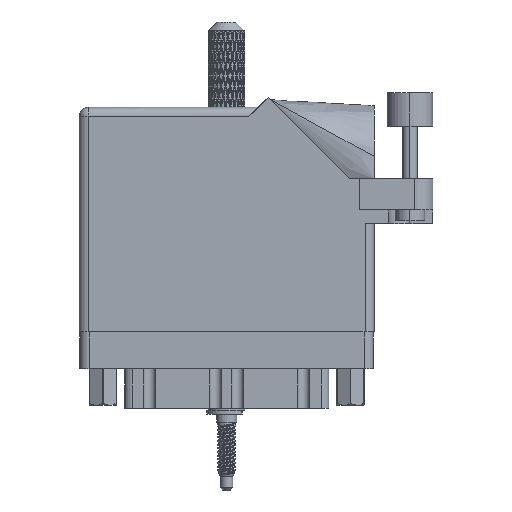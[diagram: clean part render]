
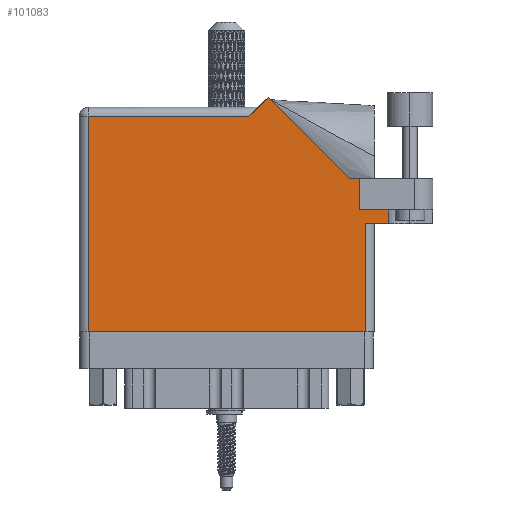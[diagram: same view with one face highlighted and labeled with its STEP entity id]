
A CAD part, front view. The second image highlights one B-rep face of the part: STEP entity #101083.
In plain terms, the highlighted face is planar.
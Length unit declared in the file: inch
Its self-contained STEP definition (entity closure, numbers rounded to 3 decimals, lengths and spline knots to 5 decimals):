
#764 = ORIENTED_EDGE ( 'NONE', *, *, #93199, .F. ) ;
#1494 = CARTESIAN_POINT ( 'NONE',  ( 0.062, 0., 0. ) ) ;
#5880 = DIRECTION ( 'NONE',  ( -1., 0., 0. ) ) ;
#8115 = ORIENTED_EDGE ( 'NONE', *, *, #74659, .T. ) ;
#10553 = CARTESIAN_POINT ( 'NONE',  ( 2.1115, 0.737, 0. ) ) ;
#10583 = VECTOR ( 'NONE', #10934, 39.37008 ) ;
#10934 = DIRECTION ( 'NONE',  ( 0., -1., 0. ) ) ;
#11982 = VERTEX_POINT ( 'NONE', #92862 ) ;
#13901 = DIRECTION ( 'NONE',  ( 1., 0., 0. ) ) ;
#15610 = VECTOR ( 'NONE', #15700, 39.37008 ) ;
#15700 = DIRECTION ( 'NONE',  ( -0.707, 0.707, 0. ) ) ;
#16142 = EDGE_CURVE ( 'NONE', #69696, #36570, #74704, .T. ) ;
#17372 = EDGE_CURVE ( 'NONE', #57398, #100621, #43704, .T. ) ;
#19483 = DIRECTION ( 'NONE',  ( -1., 0., 0. ) ) ;
#20174 = VERTEX_POINT ( 'NONE', #97081 ) ;
#22118 = CARTESIAN_POINT ( 'NONE',  ( 0.062, 0., 0. ) ) ;
#22520 = LINE ( 'NONE', #57601, #79626 ) ;
#24242 = EDGE_CURVE ( 'NONE', #81942, #102610, #106608, .T. ) ;
#27284 = DIRECTION ( 'NONE',  ( 0., -1., 0. ) ) ;
#28101 = CARTESIAN_POINT ( 'NONE',  ( 2.41, 1.044, 0. ) ) ;
#30601 = CARTESIAN_POINT ( 'NONE',  ( 1.91, 0.831, 0. ) ) ;
#32043 = ORIENTED_EDGE ( 'NONE', *, *, #16142, .T. ) ;
#32108 = EDGE_CURVE ( 'NONE', #36570, #81942, #65064, .T. ) ;
#33150 = AXIS2_PLACEMENT_3D ( 'NONE', #111329, #84917, #95279 ) ;
#36570 = VERTEX_POINT ( 'NONE', #84374 ) ;
#36747 = LINE ( 'NONE', #28101, #78238 ) ;
#38378 = ORIENTED_EDGE ( 'NONE', *, *, #86738, .F. ) ;
#40867 = CARTESIAN_POINT ( 'NONE',  ( 0., 1.468, 0. ) ) ;
#41526 = EDGE_LOOP ( 'NONE', ( #105941, #44499, #101186, #764, #38378, #53182, #8115, #90428, #32043, #53290, #87346 ) ) ;
#42484 = CARTESIAN_POINT ( 'NONE',  ( 1.91, 0.831, 0. ) ) ;
#43324 = VERTEX_POINT ( 'NONE', #94800 ) ;
#43704 = LINE ( 'NONE', #113252, #76299 ) ;
#44499 = ORIENTED_EDGE ( 'NONE', *, *, #60868, .T. ) ;
#48830 = CARTESIAN_POINT ( 'NONE',  ( 1.217, 1.53, 0. ) ) ;
#48988 = DIRECTION ( 'NONE',  ( 1., 0., 0. ) ) ;
#49410 = LINE ( 'NONE', #42484, #67772 ) ;
#49412 = VECTOR ( 'NONE', #59577, 39.37008 ) ;
#51460 = VERTEX_POINT ( 'NONE', #56876 ) ;
#53182 = ORIENTED_EDGE ( 'NONE', *, *, #87078, .T. ) ;
#53290 = ORIENTED_EDGE ( 'NONE', *, *, #32108, .T. ) ;
#56044 = CARTESIAN_POINT ( 'NONE',  ( 1.28771, 1.60071, 0. ) ) ;
#56068 = CARTESIAN_POINT ( 'NONE',  ( 2.1115, 0.831, 0. ) ) ;
#56876 = CARTESIAN_POINT ( 'NONE',  ( 1.91, 1.044, 0. ) ) ;
#57398 = VERTEX_POINT ( 'NONE', #92781 ) ;
#57601 = CARTESIAN_POINT ( 'NONE',  ( 0., 0., 0. ) ) ;
#58112 = VECTOR ( 'NONE', #27284, 39.37008 ) ;
#59577 = DIRECTION ( 'NONE',  ( 0., 1., 0. ) ) ;
#60221 = FACE_OUTER_BOUND ( 'NONE', #41526, .T. ) ;
#60868 = EDGE_CURVE ( 'NONE', #20174, #57398, #77374, .T. ) ;
#63235 = VECTOR ( 'NONE', #90836, 39.37008 ) ;
#63322 = EDGE_CURVE ( 'NONE', #102610, #20174, #22520, .T. ) ;
#65064 = LINE ( 'NONE', #40867, #99186 ) ;
#66901 = EDGE_CURVE ( 'NONE', #11982, #69696, #110541, .T. ) ;
#67772 = VECTOR ( 'NONE', #68947, 39.37008 ) ;
#68947 = DIRECTION ( 'NONE',  ( 0., 1., 0. ) ) ;
#69696 = VERTEX_POINT ( 'NONE', #56044 ) ;
#74309 = LINE ( 'NONE', #30601, #75006 ) ;
#74659 = EDGE_CURVE ( 'NONE', #51460, #11982, #36747, .T. ) ;
#74704 = LINE ( 'NONE', #48830, #63235 ) ;
#75006 = VECTOR ( 'NONE', #48988, 39.37008 ) ;
#75577 = CARTESIAN_POINT ( 'NONE',  ( 0.062, 1.468, 0. ) ) ;
#76299 = VECTOR ( 'NONE', #86272, 39.37008 ) ;
#77374 = LINE ( 'NONE', #95204, #49412 ) ;
#77448 = PLANE ( 'NONE',  #33150 ) ;
#78238 = VECTOR ( 'NONE', #19483, 39.37008 ) ;
#79626 = VECTOR ( 'NONE', #13901, 39.37008 ) ;
#81942 = VERTEX_POINT ( 'NONE', #75577 ) ;
#84374 = CARTESIAN_POINT ( 'NONE',  ( 1.155, 1.468, 0. ) ) ;
#84917 = DIRECTION ( 'NONE',  ( 0., 0., -1. ) ) ;
#86272 = DIRECTION ( 'NONE',  ( 1., 0., 0. ) ) ;
#86738 = EDGE_CURVE ( 'NONE', #43324, #110630, #74309, .T. ) ;
#87078 = EDGE_CURVE ( 'NONE', #43324, #51460, #49410, .T. ) ;
#87346 = ORIENTED_EDGE ( 'NONE', *, *, #24242, .T. ) ;
#89661 = LINE ( 'NONE', #98292, #10583 ) ;
#90428 = ORIENTED_EDGE ( 'NONE', *, *, #66901, .T. ) ;
#90836 = DIRECTION ( 'NONE',  ( -0.707, -0.707, 0. ) ) ;
#92781 = CARTESIAN_POINT ( 'NONE',  ( 1.948, 0.737, 0. ) ) ;
#92862 = CARTESIAN_POINT ( 'NONE',  ( 1.84442, 1.044, 0. ) ) ;
#93199 = EDGE_CURVE ( 'NONE', #110630, #100621, #89661, .T. ) ;
#94800 = CARTESIAN_POINT ( 'NONE',  ( 1.91, 0.831, 0. ) ) ;
#95204 = CARTESIAN_POINT ( 'NONE',  ( 1.948, 0.737, 0. ) ) ;
#95279 = DIRECTION ( 'NONE',  ( -1., 0., 0. ) ) ;
#97081 = CARTESIAN_POINT ( 'NONE',  ( 1.948, 0., 0. ) ) ;
#98292 = CARTESIAN_POINT ( 'NONE',  ( 2.1115, 1.16177, 0. ) ) ;
#99186 = VECTOR ( 'NONE', #5880, 39.37008 ) ;
#100621 = VERTEX_POINT ( 'NONE', #10553 ) ;
#101083 = ADVANCED_FACE ( 'NONE', ( #60221 ), #77448, .F. ) ;
#101186 = ORIENTED_EDGE ( 'NONE', *, *, #17372, .T. ) ;
#102508 = CARTESIAN_POINT ( 'NONE',  ( 1.84442, 1.044, 0. ) ) ;
#102610 = VERTEX_POINT ( 'NONE', #22118 ) ;
#105941 = ORIENTED_EDGE ( 'NONE', *, *, #63322, .T. ) ;
#106608 = LINE ( 'NONE', #1494, #58112 ) ;
#110541 = LINE ( 'NONE', #102508, #15610 ) ;
#110630 = VERTEX_POINT ( 'NONE', #56068 ) ;
#111329 = CARTESIAN_POINT ( 'NONE',  ( 0., 1.53, 0. ) ) ;
#113252 = CARTESIAN_POINT ( 'NONE',  ( 2.01, 0.737, 0. ) ) ;
